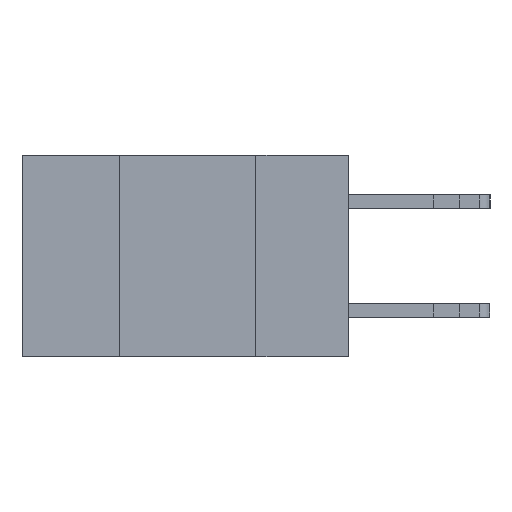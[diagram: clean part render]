
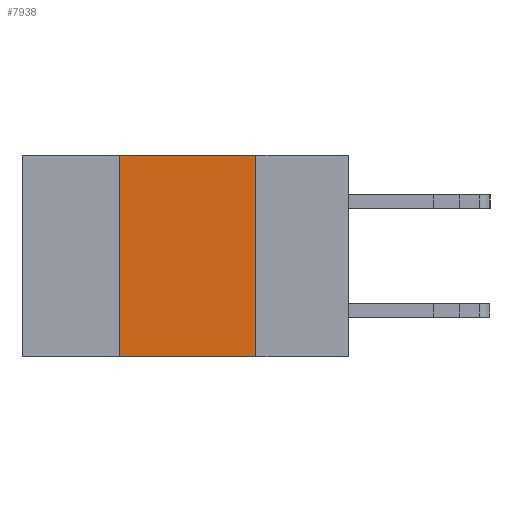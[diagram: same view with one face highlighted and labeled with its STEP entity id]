
A CAD part, left-side view. The second image highlights one B-rep face of the part: STEP entity #7938.
In plain terms, the highlighted planar face has unit normal (-1, 0, 0).
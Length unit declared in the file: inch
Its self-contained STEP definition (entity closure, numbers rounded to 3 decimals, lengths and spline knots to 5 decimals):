
#979 = FACE_OUTER_BOUND ( 'NONE', #2655, .T. ) ;
#1025 = CARTESIAN_POINT ( 'NONE',  ( 0., 0.6, -0.37 ) ) ;
#1053 = DIRECTION ( 'NONE',  ( 0., 0., 1. ) ) ;
#1716 = DIRECTION ( 'NONE',  ( 0., -1., 0. ) ) ;
#2655 = EDGE_LOOP ( 'NONE', ( #10520, #9436, #9956, #4896 ) ) ;
#3024 = CARTESIAN_POINT ( 'NONE',  ( 0., 0.6, 0. ) ) ;
#3112 = DIRECTION ( 'NONE',  ( 0., 0., -1. ) ) ;
#3327 = VERTEX_POINT ( 'NONE', #5664 ) ;
#3844 = EDGE_CURVE ( 'NONE', #3327, #8914, #9681, .T. ) ;
#3916 = DIRECTION ( 'NONE',  ( 0., 0., -1. ) ) ;
#4261 = CARTESIAN_POINT ( 'NONE',  ( 0., 0.17, -0.37 ) ) ;
#4896 = ORIENTED_EDGE ( 'NONE', *, *, #9201, .T. ) ;
#5602 = CARTESIAN_POINT ( 'NONE',  ( 0., 0.42, -0.37 ) ) ;
#5664 = CARTESIAN_POINT ( 'NONE',  ( 0., 0.17, 0. ) ) ;
#6019 = EDGE_CURVE ( 'NONE', #10638, #3327, #8805, .T. ) ;
#6167 = VECTOR ( 'NONE', #1716, 39.37008 ) ;
#6223 = LINE ( 'NONE', #1025, #10660 ) ;
#6598 = DIRECTION ( 'NONE',  ( 0., -1., 0. ) ) ;
#7157 = CARTESIAN_POINT ( 'NONE',  ( 0., 0.6, 0. ) ) ;
#7817 = AXIS2_PLACEMENT_3D ( 'NONE', #3024, #9233, #3916 ) ;
#7938 = ADVANCED_FACE ( 'NONE', ( #979 ), #8332, .F. ) ;
#7987 = EDGE_CURVE ( 'NONE', #10378, #10638, #11922, .T. ) ;
#8332 = PLANE ( 'NONE',  #7817 ) ;
#8380 = CARTESIAN_POINT ( 'NONE',  ( 0., 0.42, 0. ) ) ;
#8805 = LINE ( 'NONE', #7157, #6167 ) ;
#8914 = VERTEX_POINT ( 'NONE', #4261 ) ;
#9201 = EDGE_CURVE ( 'NONE', #10378, #8914, #6223, .T. ) ;
#9233 = DIRECTION ( 'NONE',  ( 1., 0., 0. ) ) ;
#9436 = ORIENTED_EDGE ( 'NONE', *, *, #6019, .F. ) ;
#9584 = VECTOR ( 'NONE', #1053, 39.37008 ) ;
#9681 = LINE ( 'NONE', #11133, #9951 ) ;
#9951 = VECTOR ( 'NONE', #3112, 39.37008 ) ;
#9956 = ORIENTED_EDGE ( 'NONE', *, *, #7987, .F. ) ;
#10378 = VERTEX_POINT ( 'NONE', #5602 ) ;
#10520 = ORIENTED_EDGE ( 'NONE', *, *, #3844, .F. ) ;
#10638 = VERTEX_POINT ( 'NONE', #11466 ) ;
#10660 = VECTOR ( 'NONE', #6598, 39.37008 ) ;
#11133 = CARTESIAN_POINT ( 'NONE',  ( 0., 0.17, 0. ) ) ;
#11466 = CARTESIAN_POINT ( 'NONE',  ( 0., 0.42, 0. ) ) ;
#11922 = LINE ( 'NONE', #8380, #9584 ) ;
